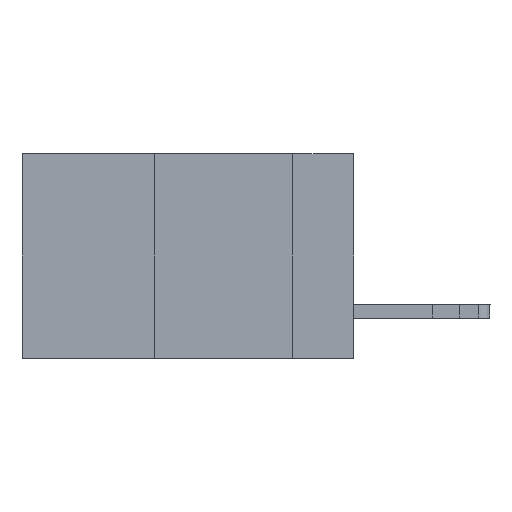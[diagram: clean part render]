
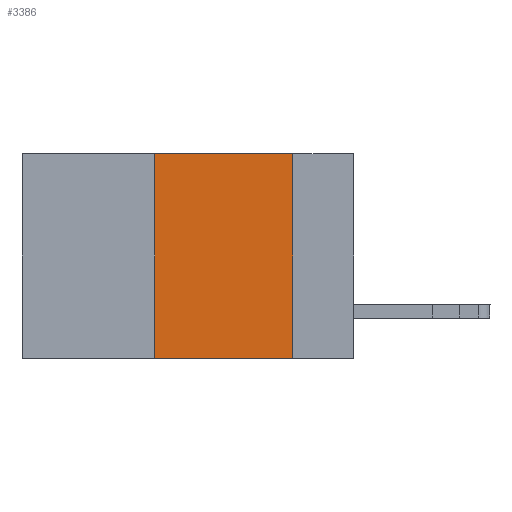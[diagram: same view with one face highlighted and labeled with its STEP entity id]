
A CAD part, left-side view. The second image highlights one B-rep face of the part: STEP entity #3386.
In plain terms, the highlighted planar face has unit normal (-1, 0, 0).
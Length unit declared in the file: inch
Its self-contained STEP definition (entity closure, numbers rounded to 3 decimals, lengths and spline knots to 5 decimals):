
#248 = LINE ( 'NONE', #12056, #8419 ) ;
#760 = CARTESIAN_POINT ( 'NONE',  ( 0., 0.6, 0. ) ) ;
#778 = VECTOR ( 'NONE', #11305, 39.37008 ) ;
#842 = ORIENTED_EDGE ( 'NONE', *, *, #2799, .T. ) ;
#1023 = LINE ( 'NONE', #8909, #12620 ) ;
#1130 = EDGE_CURVE ( 'NONE', #3298, #9937, #1023, .T. ) ;
#1152 = CARTESIAN_POINT ( 'NONE',  ( 0., 0.11, 0. ) ) ;
#1424 = VERTEX_POINT ( 'NONE', #11571 ) ;
#2064 = ORIENTED_EDGE ( 'NONE', *, *, #9599, .F. ) ;
#2799 = EDGE_CURVE ( 'NONE', #3298, #1424, #248, .T. ) ;
#2850 = DIRECTION ( 'NONE',  ( 0., 0., -1. ) ) ;
#2890 = ORIENTED_EDGE ( 'NONE', *, *, #9056, .F. ) ;
#2900 = CARTESIAN_POINT ( 'NONE',  ( 0., 0.36, -0.37 ) ) ;
#3298 = VERTEX_POINT ( 'NONE', #2900 ) ;
#3386 = ADVANCED_FACE ( 'NONE', ( #9300 ), #11101, .F. ) ;
#4322 = CARTESIAN_POINT ( 'NONE',  ( 0., 0.6, 0. ) ) ;
#5132 = DIRECTION ( 'NONE',  ( 0., -1., 0. ) ) ;
#6024 = AXIS2_PLACEMENT_3D ( 'NONE', #760, #9781, #2850 ) ;
#6360 = CARTESIAN_POINT ( 'NONE',  ( 0., 0.36, 0. ) ) ;
#7922 = EDGE_LOOP ( 'NONE', ( #2890, #2064, #9953, #842 ) ) ;
#8063 = LINE ( 'NONE', #10293, #13315 ) ;
#8419 = VECTOR ( 'NONE', #5132, 39.37008 ) ;
#8909 = CARTESIAN_POINT ( 'NONE',  ( 0., 0.36, 0. ) ) ;
#9002 = DIRECTION ( 'NONE',  ( 0., 0., 1. ) ) ;
#9056 = EDGE_CURVE ( 'NONE', #14306, #1424, #8063, .T. ) ;
#9300 = FACE_OUTER_BOUND ( 'NONE', #7922, .T. ) ;
#9599 = EDGE_CURVE ( 'NONE', #9937, #14306, #10941, .T. ) ;
#9781 = DIRECTION ( 'NONE',  ( 1., 0., 0. ) ) ;
#9937 = VERTEX_POINT ( 'NONE', #6360 ) ;
#9953 = ORIENTED_EDGE ( 'NONE', *, *, #1130, .F. ) ;
#10293 = CARTESIAN_POINT ( 'NONE',  ( 0., 0.11, 0. ) ) ;
#10941 = LINE ( 'NONE', #4322, #778 ) ;
#11101 = PLANE ( 'NONE',  #6024 ) ;
#11305 = DIRECTION ( 'NONE',  ( 0., -1., 0. ) ) ;
#11553 = DIRECTION ( 'NONE',  ( 0., 0., -1. ) ) ;
#11571 = CARTESIAN_POINT ( 'NONE',  ( 0., 0.11, -0.37 ) ) ;
#12056 = CARTESIAN_POINT ( 'NONE',  ( 0., 0.6, -0.37 ) ) ;
#12620 = VECTOR ( 'NONE', #9002, 39.37008 ) ;
#13315 = VECTOR ( 'NONE', #11553, 39.37008 ) ;
#14306 = VERTEX_POINT ( 'NONE', #1152 ) ;
